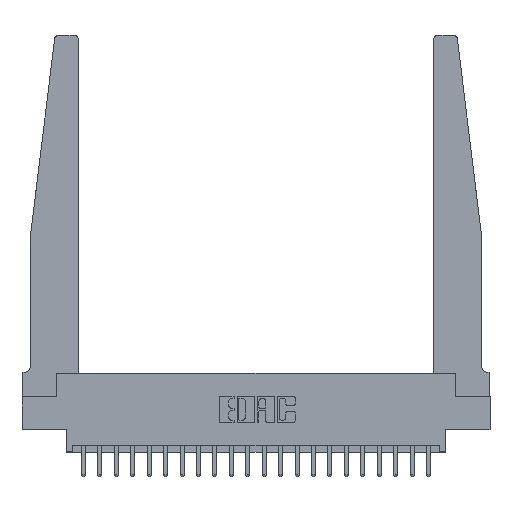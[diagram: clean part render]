
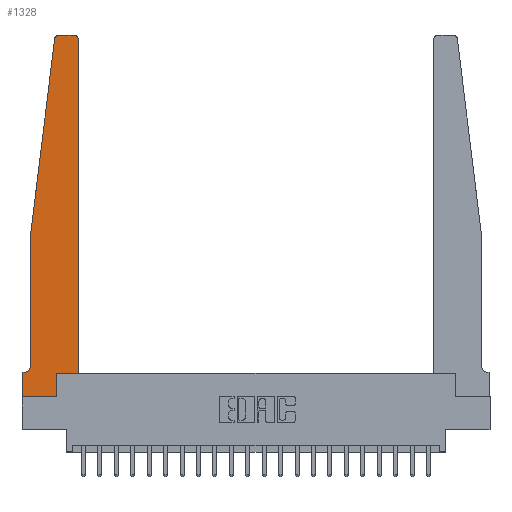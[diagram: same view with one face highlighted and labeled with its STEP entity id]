
A CAD part, top view. The second image highlights one B-rep face of the part: STEP entity #1328.
In plain terms, the highlighted planar face has unit normal (0, 0, 1).
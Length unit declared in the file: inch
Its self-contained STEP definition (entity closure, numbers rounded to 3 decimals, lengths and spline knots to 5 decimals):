
#698 = ORIENTED_EDGE ( 'NONE', *, *, #2774, .T. ) ;
#1110 = LINE ( 'NONE', #21948, #14341 ) ;
#1328 = ADVANCED_FACE ( 'NONE', ( #10593 ), #15681, .T. ) ;
#1493 = DIRECTION ( 'NONE',  ( 0., 0., -1. ) ) ;
#1673 = EDGE_CURVE ( 'NONE', #13054, #15223, #16189, .T. ) ;
#1803 = DIRECTION ( 'NONE',  ( 1., 0., 0. ) ) ;
#2058 = CARTESIAN_POINT ( 'NONE',  ( 0.25, 2.75, 0.37 ) ) ;
#2115 = EDGE_CURVE ( 'NONE', #12692, #18279, #17014, .T. ) ;
#2148 = VERTEX_POINT ( 'NONE', #5993 ) ;
#2774 = EDGE_CURVE ( 'NONE', #8515, #13054, #1110, .T. ) ;
#2954 = LINE ( 'NONE', #2058, #16627 ) ;
#3082 = EDGE_LOOP ( 'NONE', ( #10353, #13972, #16555, #5205, #19126, #6444, #18006, #16787, #3234, #698, #17349, #14327 ) ) ;
#3234 = ORIENTED_EDGE ( 'NONE', *, *, #11543, .T. ) ;
#3369 = CARTESIAN_POINT ( 'NONE',  ( 0.2605, 0.18, 0.37 ) ) ;
#3806 = DIRECTION ( 'NONE',  ( -1., 0., 0. ) ) ;
#4945 = EDGE_CURVE ( 'NONE', #11305, #17984, #2954, .T. ) ;
#5130 = DIRECTION ( 'NONE',  ( 0., 1., 0. ) ) ;
#5205 = ORIENTED_EDGE ( 'NONE', *, *, #2115, .T. ) ;
#5299 = CARTESIAN_POINT ( 'NONE',  ( 0., 0., 0.37 ) ) ;
#5324 = VERTEX_POINT ( 'NONE', #16819 ) ;
#5770 = EDGE_CURVE ( 'NONE', #15223, #11305, #19252, .T. ) ;
#5780 = CARTESIAN_POINT ( 'NONE',  ( 0.27653, 2.72, 0.37 ) ) ;
#5983 = CARTESIAN_POINT ( 'NONE',  ( 0.2605, 0.18, 0.37 ) ) ;
#5993 = CARTESIAN_POINT ( 'NONE',  ( 0., 0.1875, 0.37 ) ) ;
#6134 = LINE ( 'NONE', #9962, #10567 ) ;
#6444 = ORIENTED_EDGE ( 'NONE', *, *, #10393, .T. ) ;
#6539 = CARTESIAN_POINT ( 'NONE',  ( 0.065, 1.25, 0.37 ) ) ;
#6547 = CIRCLE ( 'NONE', #21658, 0.03 ) ;
#6665 = DIRECTION ( 'NONE',  ( 0., -1., 0. ) ) ;
#7048 = VECTOR ( 'NONE', #8190, 39.37008 ) ;
#7489 = DIRECTION ( 'NONE',  ( 1., 0., 0. ) ) ;
#7801 = EDGE_CURVE ( 'NONE', #17984, #18677, #6547, .T. ) ;
#8160 = CIRCLE ( 'NONE', #9252, 0.05 ) ;
#8190 = DIRECTION ( 'NONE',  ( -1., 0., 0. ) ) ;
#8264 = EDGE_CURVE ( 'NONE', #2148, #11016, #21126, .T. ) ;
#8323 = CARTESIAN_POINT ( 'NONE',  ( 0.425, 0.18, 0.37 ) ) ;
#8459 = VECTOR ( 'NONE', #6665, 39.37008 ) ;
#8515 = VERTEX_POINT ( 'NONE', #5983 ) ;
#9174 = CARTESIAN_POINT ( 'NONE',  ( 0.065, 1.25, 0.37 ) ) ;
#9252 = AXIS2_PLACEMENT_3D ( 'NONE', #11824, #1493, #13530 ) ;
#9711 = CARTESIAN_POINT ( 'NONE',  ( 0.395, 2.72, 0.37 ) ) ;
#9962 = CARTESIAN_POINT ( 'NONE',  ( 0.065, 1.25, 0.37 ) ) ;
#10353 = ORIENTED_EDGE ( 'NONE', *, *, #4945, .T. ) ;
#10393 = EDGE_CURVE ( 'NONE', #19437, #2148, #19574, .T. ) ;
#10567 = VECTOR ( 'NONE', #11680, 39.37008 ) ;
#10593 = FACE_OUTER_BOUND ( 'NONE', #3082, .T. ) ;
#11016 = VERTEX_POINT ( 'NONE', #5299 ) ;
#11305 = VERTEX_POINT ( 'NONE', #19646 ) ;
#11412 = DIRECTION ( 'NONE',  ( 1., 0., 0. ) ) ;
#11543 = EDGE_CURVE ( 'NONE', #5324, #8515, #12573, .T. ) ;
#11637 = DIRECTION ( 'NONE',  ( 0., 1., 0. ) ) ;
#11648 = VECTOR ( 'NONE', #11637, 39.37008 ) ;
#11680 = DIRECTION ( 'NONE',  ( -0.122, -0.992, 0. ) ) ;
#11824 = CARTESIAN_POINT ( 'NONE',  ( 0.015, 0.2375, 0.37 ) ) ;
#11834 = CARTESIAN_POINT ( 'NONE',  ( 0.425, 0.18, 0.37 ) ) ;
#11843 = CARTESIAN_POINT ( 'NONE',  ( 0., 0., 0.37 ) ) ;
#11892 = CARTESIAN_POINT ( 'NONE',  ( 0.425, 2.72, 0.37 ) ) ;
#12025 = VECTOR ( 'NONE', #5130, 39.37008 ) ;
#12140 = EDGE_CURVE ( 'NONE', #11016, #5324, #18922, .T. ) ;
#12177 = VECTOR ( 'NONE', #13546, 39.37008 ) ;
#12467 = CARTESIAN_POINT ( 'NONE',  ( 0., 0., 0.37 ) ) ;
#12573 = LINE ( 'NONE', #3369, #12025 ) ;
#12692 = VERTEX_POINT ( 'NONE', #9174 ) ;
#12998 = EDGE_CURVE ( 'NONE', #18677, #12692, #6134, .T. ) ;
#13054 = VERTEX_POINT ( 'NONE', #8323 ) ;
#13530 = DIRECTION ( 'NONE',  ( -1., 0., 0. ) ) ;
#13546 = DIRECTION ( 'NONE',  ( 0., -1., 0. ) ) ;
#13972 = ORIENTED_EDGE ( 'NONE', *, *, #7801, .T. ) ;
#14012 = CARTESIAN_POINT ( 'NONE',  ( 0.015, 0.1875, 0.37 ) ) ;
#14201 = DIRECTION ( 'NONE',  ( 1., 0., 0. ) ) ;
#14327 = ORIENTED_EDGE ( 'NONE', *, *, #5770, .T. ) ;
#14341 = VECTOR ( 'NONE', #1803, 39.37008 ) ;
#14939 = VECTOR ( 'NONE', #14201, 39.37008 ) ;
#15097 = CARTESIAN_POINT ( 'NONE',  ( 0.27653, 2.75, 0.37 ) ) ;
#15223 = VERTEX_POINT ( 'NONE', #11892 ) ;
#15535 = DIRECTION ( 'NONE',  ( 1., 0., 0. ) ) ;
#15580 = DIRECTION ( 'NONE',  ( 0., 0., 1. ) ) ;
#15626 = CARTESIAN_POINT ( 'NONE',  ( 0., 0.1875, 0.37 ) ) ;
#15681 = PLANE ( 'NONE',  #19951 ) ;
#16189 = LINE ( 'NONE', #11834, #11648 ) ;
#16555 = ORIENTED_EDGE ( 'NONE', *, *, #12998, .T. ) ;
#16627 = VECTOR ( 'NONE', #3806, 39.37008 ) ;
#16787 = ORIENTED_EDGE ( 'NONE', *, *, #12140, .T. ) ;
#16819 = CARTESIAN_POINT ( 'NONE',  ( 0.2605, 0., 0.37 ) ) ;
#17014 = LINE ( 'NONE', #6539, #8459 ) ;
#17349 = ORIENTED_EDGE ( 'NONE', *, *, #1673, .T. ) ;
#17742 = DIRECTION ( 'NONE',  ( 0., 0., 1. ) ) ;
#17984 = VERTEX_POINT ( 'NONE', #15097 ) ;
#18006 = ORIENTED_EDGE ( 'NONE', *, *, #8264, .T. ) ;
#18279 = VERTEX_POINT ( 'NONE', #19256 ) ;
#18418 = CARTESIAN_POINT ( 'NONE',  ( 0.065, 0.1875, 0.37 ) ) ;
#18624 = AXIS2_PLACEMENT_3D ( 'NONE', #9711, #21529, #11412 ) ;
#18677 = VERTEX_POINT ( 'NONE', #18795 ) ;
#18795 = CARTESIAN_POINT ( 'NONE',  ( 0.24675, 2.72367, 0.37 ) ) ;
#18922 = LINE ( 'NONE', #12467, #14939 ) ;
#19126 = ORIENTED_EDGE ( 'NONE', *, *, #21583, .T. ) ;
#19252 = CIRCLE ( 'NONE', #18624, 0.03 ) ;
#19256 = CARTESIAN_POINT ( 'NONE',  ( 0.065, 0.2375, 0.37 ) ) ;
#19437 = VERTEX_POINT ( 'NONE', #14012 ) ;
#19574 = LINE ( 'NONE', #18418, #7048 ) ;
#19646 = CARTESIAN_POINT ( 'NONE',  ( 0.395, 2.75, 0.37 ) ) ;
#19951 = AXIS2_PLACEMENT_3D ( 'NONE', #15626, #15580, #15535 ) ;
#21126 = LINE ( 'NONE', #11843, #12177 ) ;
#21529 = DIRECTION ( 'NONE',  ( 0., 0., 1. ) ) ;
#21583 = EDGE_CURVE ( 'NONE', #18279, #19437, #8160, .T. ) ;
#21658 = AXIS2_PLACEMENT_3D ( 'NONE', #5780, #17742, #7489 ) ;
#21948 = CARTESIAN_POINT ( 'NONE',  ( 0.425, 0.18, 0.37 ) ) ;
